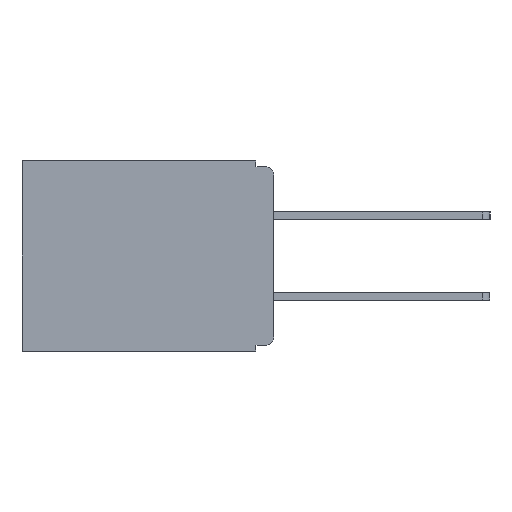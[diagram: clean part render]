
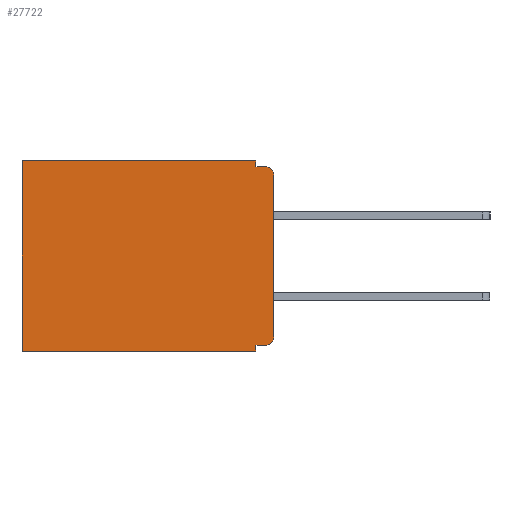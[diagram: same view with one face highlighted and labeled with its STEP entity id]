
A CAD part, left-side view. The second image highlights one B-rep face of the part: STEP entity #27722.
In plain terms, the highlighted planar face has unit normal (-1, 0, 0).
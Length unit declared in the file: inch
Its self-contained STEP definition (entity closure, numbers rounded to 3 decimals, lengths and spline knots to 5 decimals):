
#458 = DIRECTION ( 'NONE',  ( 0., 0., -1. ) ) ;
#825 = VERTEX_POINT ( 'NONE', #28967 ) ;
#910 = LINE ( 'NONE', #17954, #17671 ) ;
#1458 = CARTESIAN_POINT ( 'NONE',  ( 0.3, 0.031, -0.01 ) ) ;
#1509 = PLANE ( 'NONE',  #8412 ) ;
#1748 = EDGE_CURVE ( 'NONE', #31778, #7014, #12270, .T. ) ;
#1840 = EDGE_CURVE ( 'NONE', #4679, #8831, #16717, .T. ) ;
#2286 = ORIENTED_EDGE ( 'NONE', *, *, #21478, .F. ) ;
#2535 = LINE ( 'NONE', #21152, #14757 ) ;
#2879 = VECTOR ( 'NONE', #17388, 39.37008 ) ;
#3055 = CARTESIAN_POINT ( 'NONE',  ( 0.3, 0.031, 0. ) ) ;
#3298 = DIRECTION ( 'NONE',  ( 0., 0., -1. ) ) ;
#3467 = CARTESIAN_POINT ( 'NONE',  ( 0.3, 0., -0.33 ) ) ;
#3811 = VERTEX_POINT ( 'NONE', #16364 ) ;
#4525 = EDGE_CURVE ( 'NONE', #12171, #4679, #24118, .T. ) ;
#4679 = VERTEX_POINT ( 'NONE', #1458 ) ;
#4839 = ORIENTED_EDGE ( 'NONE', *, *, #1840, .F. ) ;
#5297 = VERTEX_POINT ( 'NONE', #23559 ) ;
#5386 = VECTOR ( 'NONE', #32900, 39.37008 ) ;
#6181 = EDGE_CURVE ( 'NONE', #20657, #3811, #12126, .T. ) ;
#6339 = DIRECTION ( 'NONE',  ( -1., 0., 0. ) ) ;
#6471 = ORIENTED_EDGE ( 'NONE', *, *, #6181, .F. ) ;
#6860 = DIRECTION ( 'NONE',  ( 0., 0., -1. ) ) ;
#7014 = VERTEX_POINT ( 'NONE', #17106 ) ;
#8412 = AXIS2_PLACEMENT_3D ( 'NONE', #19736, #22270, #6860 ) ;
#8501 = ORIENTED_EDGE ( 'NONE', *, *, #13837, .T. ) ;
#8610 = CIRCLE ( 'NONE', #28184, 0.015 ) ;
#8831 = VERTEX_POINT ( 'NONE', #25025 ) ;
#9071 = DIRECTION ( 'NONE',  ( 0., 0., -1. ) ) ;
#9100 = FACE_OUTER_BOUND ( 'NONE', #29981, .T. ) ;
#9144 = EDGE_CURVE ( 'NONE', #5297, #3811, #24311, .T. ) ;
#9172 = CARTESIAN_POINT ( 'NONE',  ( 0.3, 0.031, 0. ) ) ;
#10111 = ORIENTED_EDGE ( 'NONE', *, *, #22718, .T. ) ;
#11661 = VECTOR ( 'NONE', #19113, 39.37008 ) ;
#12126 = LINE ( 'NONE', #28962, #24955 ) ;
#12171 = VERTEX_POINT ( 'NONE', #3055 ) ;
#12270 = LINE ( 'NONE', #3467, #5386 ) ;
#12750 = DIRECTION ( 'NONE',  ( 0., 1., 0. ) ) ;
#13837 = EDGE_CURVE ( 'NONE', #12171, #15303, #910, .T. ) ;
#14757 = VECTOR ( 'NONE', #28807, 39.37008 ) ;
#15222 = CARTESIAN_POINT ( 'NONE',  ( 0.3, 0., -0.025 ) ) ;
#15303 = VERTEX_POINT ( 'NONE', #21241 ) ;
#16125 = DIRECTION ( 'NONE',  ( -1., 0., 0. ) ) ;
#16364 = CARTESIAN_POINT ( 'NONE',  ( 0.3, 0., -0.305 ) ) ;
#16717 = LINE ( 'NONE', #32452, #2879 ) ;
#17106 = CARTESIAN_POINT ( 'NONE',  ( 0.3, 0.437, -0.33 ) ) ;
#17349 = VECTOR ( 'NONE', #9071, 39.37008 ) ;
#17358 = ORIENTED_EDGE ( 'NONE', *, *, #9144, .T. ) ;
#17388 = DIRECTION ( 'NONE',  ( 0., -1., 0. ) ) ;
#17671 = VECTOR ( 'NONE', #12750, 39.37008 ) ;
#17954 = CARTESIAN_POINT ( 'NONE',  ( 0.3, 0., 0. ) ) ;
#18084 = AXIS2_PLACEMENT_3D ( 'NONE', #21788, #6339, #24326 ) ;
#18536 = LINE ( 'NONE', #29227, #11661 ) ;
#18669 = EDGE_CURVE ( 'NONE', #15303, #7014, #18536, .T. ) ;
#19113 = DIRECTION ( 'NONE',  ( 0., 0., -1. ) ) ;
#19736 = CARTESIAN_POINT ( 'NONE',  ( 0.3, 0., -0.33 ) ) ;
#19808 = ORIENTED_EDGE ( 'NONE', *, *, #4525, .F. ) ;
#20657 = VERTEX_POINT ( 'NONE', #15222 ) ;
#21152 = CARTESIAN_POINT ( 'NONE',  ( 0.3, 0., -0.32 ) ) ;
#21241 = CARTESIAN_POINT ( 'NONE',  ( 0.3, 0.437, 0. ) ) ;
#21478 = EDGE_CURVE ( 'NONE', #5297, #825, #2535, .T. ) ;
#21788 = CARTESIAN_POINT ( 'NONE',  ( 0.3, 0.015, -0.305 ) ) ;
#22270 = DIRECTION ( 'NONE',  ( 1., 0., 0. ) ) ;
#22718 = EDGE_CURVE ( 'NONE', #20657, #8831, #8610, .T. ) ;
#23559 = CARTESIAN_POINT ( 'NONE',  ( 0.3, 0.015, -0.32 ) ) ;
#24008 = VECTOR ( 'NONE', #24645, 39.37008 ) ;
#24118 = LINE ( 'NONE', #9172, #17349 ) ;
#24311 = CIRCLE ( 'NONE', #18084, 0.015 ) ;
#24326 = DIRECTION ( 'NONE',  ( 0., 0., -1. ) ) ;
#24645 = DIRECTION ( 'NONE',  ( 0., 0., -1. ) ) ;
#24955 = VECTOR ( 'NONE', #3298, 39.37008 ) ;
#25025 = CARTESIAN_POINT ( 'NONE',  ( 0.3, 0.015, -0.01 ) ) ;
#27031 = EDGE_CURVE ( 'NONE', #825, #31778, #30755, .T. ) ;
#27722 = ADVANCED_FACE ( 'NONE', ( #9100 ), #1509, .F. ) ;
#28184 = AXIS2_PLACEMENT_3D ( 'NONE', #31348, #16125, #458 ) ;
#28807 = DIRECTION ( 'NONE',  ( 0., 1., 0. ) ) ;
#28962 = CARTESIAN_POINT ( 'NONE',  ( 0.3, 0., -0.33 ) ) ;
#28967 = CARTESIAN_POINT ( 'NONE',  ( 0.3, 0.031, -0.32 ) ) ;
#29227 = CARTESIAN_POINT ( 'NONE',  ( 0.3, 0.437, -0.33 ) ) ;
#29981 = EDGE_LOOP ( 'NONE', ( #6471, #10111, #4839, #19808, #8501, #32040, #30104, #33186, #2286, #17358 ) ) ;
#30104 = ORIENTED_EDGE ( 'NONE', *, *, #1748, .F. ) ;
#30755 = LINE ( 'NONE', #32134, #24008 ) ;
#31348 = CARTESIAN_POINT ( 'NONE',  ( 0.3, 0.015, -0.025 ) ) ;
#31778 = VERTEX_POINT ( 'NONE', #32096 ) ;
#32040 = ORIENTED_EDGE ( 'NONE', *, *, #18669, .T. ) ;
#32096 = CARTESIAN_POINT ( 'NONE',  ( 0.3, 0.031, -0.33 ) ) ;
#32134 = CARTESIAN_POINT ( 'NONE',  ( 0.3, 0.031, -0.33 ) ) ;
#32452 = CARTESIAN_POINT ( 'NONE',  ( 0.3, 0., -0.01 ) ) ;
#32900 = DIRECTION ( 'NONE',  ( 0., 1., 0. ) ) ;
#33186 = ORIENTED_EDGE ( 'NONE', *, *, #27031, .F. ) ;
